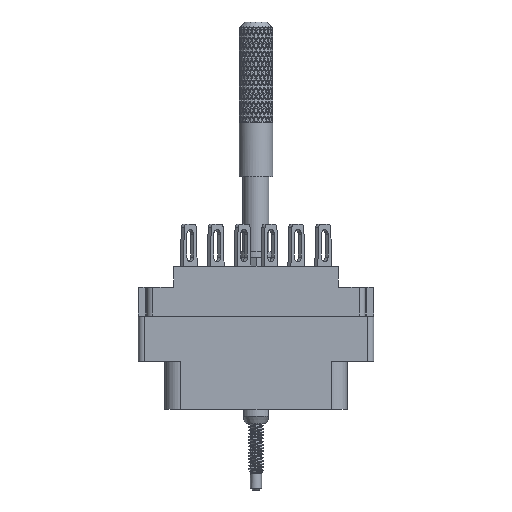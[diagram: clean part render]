
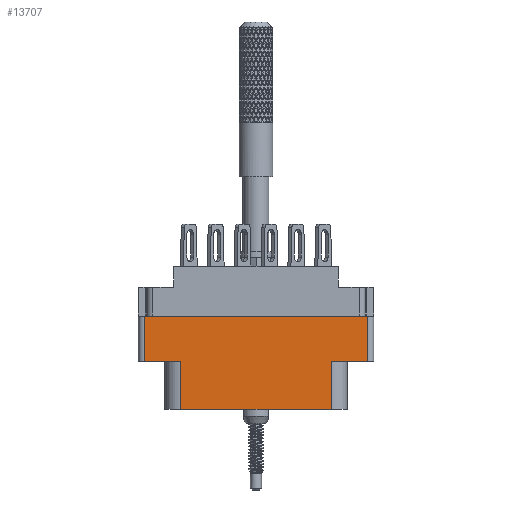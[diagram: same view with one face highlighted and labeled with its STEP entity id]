
A CAD part, front view. The second image highlights one B-rep face of the part: STEP entity #13707.
In plain terms, the highlighted planar face has unit normal (0, -1, 0).
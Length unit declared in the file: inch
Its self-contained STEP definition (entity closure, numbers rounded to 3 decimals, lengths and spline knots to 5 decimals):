
#3793 = EDGE_CURVE ( 'NONE', #112547, #104506, #16185, .T. ) ;
#4620 = EDGE_CURVE ( 'NONE', #46968, #166313, #47357, .T. ) ;
#7211 = EDGE_LOOP ( 'NONE', ( #149046, #8707, #171894, #22607, #40367, #56734, #34355, #42247 ) ) ;
#8707 = ORIENTED_EDGE ( 'NONE', *, *, #117025, .T. ) ;
#9487 = VERTEX_POINT ( 'NONE', #107600 ) ;
#13707 = ADVANCED_FACE ( 'NONE', ( #19960 ), #68690, .T. ) ;
#14766 = DIRECTION ( 'NONE',  ( 0., 0., -1. ) ) ;
#16185 = LINE ( 'NONE', #97545, #164770 ) ;
#19960 = FACE_OUTER_BOUND ( 'NONE', #7211, .T. ) ;
#19990 = AXIS2_PLACEMENT_3D ( 'NONE', #128821, #113373, #14766 ) ;
#20426 = CARTESIAN_POINT ( 'NONE',  ( -0.624, -0.343, -0.277 ) ) ;
#22607 = ORIENTED_EDGE ( 'NONE', *, *, #52760, .F. ) ;
#34355 = ORIENTED_EDGE ( 'NONE', *, *, #163275, .F. ) ;
#36130 = CARTESIAN_POINT ( 'NONE',  ( 0.42, -0.343, -0.529 ) ) ;
#36898 = EDGE_CURVE ( 'NONE', #9487, #166313, #63128, .T. ) ;
#40367 = ORIENTED_EDGE ( 'NONE', *, *, #36898, .T. ) ;
#42175 = CARTESIAN_POINT ( 'NONE',  ( 0.42, -0.343, -0.529 ) ) ;
#42247 = ORIENTED_EDGE ( 'NONE', *, *, #3793, .T. ) ;
#46952 = EDGE_CURVE ( 'NONE', #104506, #47761, #90270, .T. ) ;
#46968 = VERTEX_POINT ( 'NONE', #20426 ) ;
#47357 = LINE ( 'NONE', #58061, #180220 ) ;
#47761 = VERTEX_POINT ( 'NONE', #162595 ) ;
#49652 = VECTOR ( 'NONE', #174601, 39.37008 ) ;
#52760 = EDGE_CURVE ( 'NONE', #9487, #63399, #106145, .T. ) ;
#56734 = ORIENTED_EDGE ( 'NONE', *, *, #4620, .F. ) ;
#58061 = CARTESIAN_POINT ( 'NONE',  ( -0.656, -0.343, -0.277 ) ) ;
#63128 = LINE ( 'NONE', #133230, #116317 ) ;
#63399 = VERTEX_POINT ( 'NONE', #36130 ) ;
#64482 = DIRECTION ( 'NONE',  ( 1., 0., 0. ) ) ;
#68690 = PLANE ( 'NONE',  #19990 ) ;
#70746 = CARTESIAN_POINT ( 'NONE',  ( -0.624, -0.343, -0.529 ) ) ;
#79794 = LINE ( 'NONE', #42175, #128707 ) ;
#90270 = LINE ( 'NONE', #109857, #145748 ) ;
#93033 = DIRECTION ( 'NONE',  ( -1., 0., 0. ) ) ;
#94363 = DIRECTION ( 'NONE',  ( 0., 0., -1. ) ) ;
#97545 = CARTESIAN_POINT ( 'NONE',  ( 0., -0.343, -0.529 ) ) ;
#104506 = VERTEX_POINT ( 'NONE', #162160 ) ;
#106145 = LINE ( 'NONE', #108534, #121590 ) ;
#107600 = CARTESIAN_POINT ( 'NONE',  ( 0.624, -0.343, -0.529 ) ) ;
#108534 = CARTESIAN_POINT ( 'NONE',  ( 0., -0.343, -0.529 ) ) ;
#109857 = CARTESIAN_POINT ( 'NONE',  ( -0.42, -0.343, -0.529 ) ) ;
#112547 = VERTEX_POINT ( 'NONE', #70746 ) ;
#113373 = DIRECTION ( 'NONE',  ( 0., -1., 0. ) ) ;
#114094 = LINE ( 'NONE', #160990, #49652 ) ;
#116317 = VECTOR ( 'NONE', #175954, 39.37008 ) ;
#117025 = EDGE_CURVE ( 'NONE', #47761, #182244, #170286, .T. ) ;
#121590 = VECTOR ( 'NONE', #93033, 39.37008 ) ;
#124665 = CARTESIAN_POINT ( 'NONE',  ( 0.42, -0.343, -0.798 ) ) ;
#128707 = VECTOR ( 'NONE', #141387, 39.37008 ) ;
#128821 = CARTESIAN_POINT ( 'NONE',  ( -0.624, -0.343, -0.798 ) ) ;
#133230 = CARTESIAN_POINT ( 'NONE',  ( 0.624, -0.343, -0.798 ) ) ;
#140340 = DIRECTION ( 'NONE',  ( 1., 0., 0. ) ) ;
#141387 = DIRECTION ( 'NONE',  ( 0., 0., -1. ) ) ;
#145748 = VECTOR ( 'NONE', #94363, 39.37008 ) ;
#148111 = VECTOR ( 'NONE', #64482, 39.37008 ) ;
#149046 = ORIENTED_EDGE ( 'NONE', *, *, #46952, .T. ) ;
#150693 = CARTESIAN_POINT ( 'NONE',  ( -0.624, -0.343, -0.798 ) ) ;
#158557 = DIRECTION ( 'NONE',  ( 1., 0., 0. ) ) ;
#160990 = CARTESIAN_POINT ( 'NONE',  ( -0.624, -0.343, -0.798 ) ) ;
#162160 = CARTESIAN_POINT ( 'NONE',  ( -0.42, -0.343, -0.529 ) ) ;
#162595 = CARTESIAN_POINT ( 'NONE',  ( -0.42, -0.343, -0.798 ) ) ;
#163275 = EDGE_CURVE ( 'NONE', #112547, #46968, #114094, .T. ) ;
#164720 = CARTESIAN_POINT ( 'NONE',  ( 0.624, -0.343, -0.277 ) ) ;
#164770 = VECTOR ( 'NONE', #140340, 39.37008 ) ;
#166313 = VERTEX_POINT ( 'NONE', #164720 ) ;
#168061 = EDGE_CURVE ( 'NONE', #63399, #182244, #79794, .T. ) ;
#170286 = LINE ( 'NONE', #150693, #148111 ) ;
#171894 = ORIENTED_EDGE ( 'NONE', *, *, #168061, .F. ) ;
#174601 = DIRECTION ( 'NONE',  ( 0., 0., 1. ) ) ;
#175954 = DIRECTION ( 'NONE',  ( 0., 0., 1. ) ) ;
#180220 = VECTOR ( 'NONE', #158557, 39.37008 ) ;
#182244 = VERTEX_POINT ( 'NONE', #124665 ) ;
